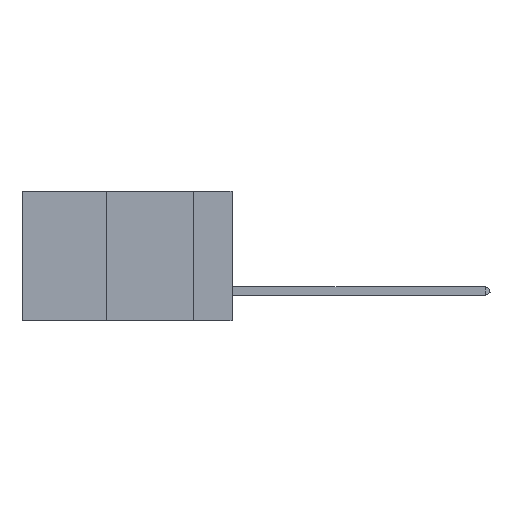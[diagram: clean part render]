
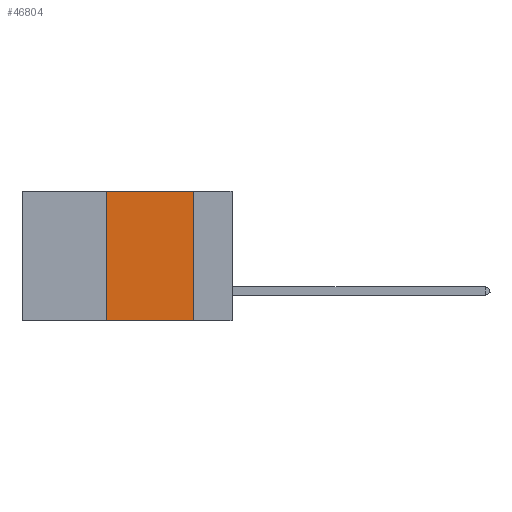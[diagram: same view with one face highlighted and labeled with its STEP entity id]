
A CAD part, left-side view. The second image highlights one B-rep face of the part: STEP entity #46804.
In plain terms, the highlighted planar face has unit normal (-1, 0, 0).
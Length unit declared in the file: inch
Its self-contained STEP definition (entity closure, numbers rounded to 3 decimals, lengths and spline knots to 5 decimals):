
#4845 = DIRECTION ( 'NONE',  ( 0., 0., 1. ) ) ;
#6573 = DIRECTION ( 'NONE',  ( 0., -1., 0. ) ) ;
#8188 = VECTOR ( 'NONE', #32859, 39.37008 ) ;
#8387 = ORIENTED_EDGE ( 'NONE', *, *, #40474, .T. ) ;
#9995 = AXIS2_PLACEMENT_3D ( 'NONE', #41960, #12921, #31379 ) ;
#11289 = LINE ( 'NONE', #25929, #8188 ) ;
#11719 = EDGE_CURVE ( 'NONE', #34488, #34332, #11289, .T. ) ;
#12090 = ORIENTED_EDGE ( 'NONE', *, *, #25008, .F. ) ;
#12921 = DIRECTION ( 'NONE',  ( 1., 0., 0. ) ) ;
#14672 = CARTESIAN_POINT ( 'NONE',  ( 0., 0.36, 0. ) ) ;
#15487 = CARTESIAN_POINT ( 'NONE',  ( 0., 0.11, -0.37 ) ) ;
#18333 = LINE ( 'NONE', #35813, #33432 ) ;
#23481 = VECTOR ( 'NONE', #6573, 39.37008 ) ;
#25008 = EDGE_CURVE ( 'NONE', #42137, #34488, #29138, .T. ) ;
#25052 = CARTESIAN_POINT ( 'NONE',  ( 0., 0.6, 0. ) ) ;
#25929 = CARTESIAN_POINT ( 'NONE',  ( 0., 0.11, 0. ) ) ;
#26688 = CARTESIAN_POINT ( 'NONE',  ( 0., 0.36, 0. ) ) ;
#27191 = ORIENTED_EDGE ( 'NONE', *, *, #35976, .F. ) ;
#27903 = VECTOR ( 'NONE', #4845, 39.37008 ) ;
#29138 = LINE ( 'NONE', #25052, #23481 ) ;
#29990 = FACE_OUTER_BOUND ( 'NONE', #41112, .T. ) ;
#31379 = DIRECTION ( 'NONE',  ( 0., 0., -1. ) ) ;
#32212 = DIRECTION ( 'NONE',  ( 0., -1., 0. ) ) ;
#32859 = DIRECTION ( 'NONE',  ( 0., 0., -1. ) ) ;
#33432 = VECTOR ( 'NONE', #32212, 39.37008 ) ;
#34332 = VERTEX_POINT ( 'NONE', #15487 ) ;
#34488 = VERTEX_POINT ( 'NONE', #34631 ) ;
#34631 = CARTESIAN_POINT ( 'NONE',  ( 0., 0.11, 0. ) ) ;
#35813 = CARTESIAN_POINT ( 'NONE',  ( 0., 0.6, -0.37 ) ) ;
#35976 = EDGE_CURVE ( 'NONE', #42188, #42137, #37258, .T. ) ;
#37258 = LINE ( 'NONE', #26688, #27903 ) ;
#39834 = ORIENTED_EDGE ( 'NONE', *, *, #11719, .F. ) ;
#40106 = CARTESIAN_POINT ( 'NONE',  ( 0., 0.36, -0.37 ) ) ;
#40474 = EDGE_CURVE ( 'NONE', #42188, #34332, #18333, .T. ) ;
#41112 = EDGE_LOOP ( 'NONE', ( #39834, #12090, #27191, #8387 ) ) ;
#41960 = CARTESIAN_POINT ( 'NONE',  ( 0., 0.6, 0. ) ) ;
#42137 = VERTEX_POINT ( 'NONE', #14672 ) ;
#42188 = VERTEX_POINT ( 'NONE', #40106 ) ;
#44637 = PLANE ( 'NONE',  #9995 ) ;
#46804 = ADVANCED_FACE ( 'NONE', ( #29990 ), #44637, .F. ) ;
